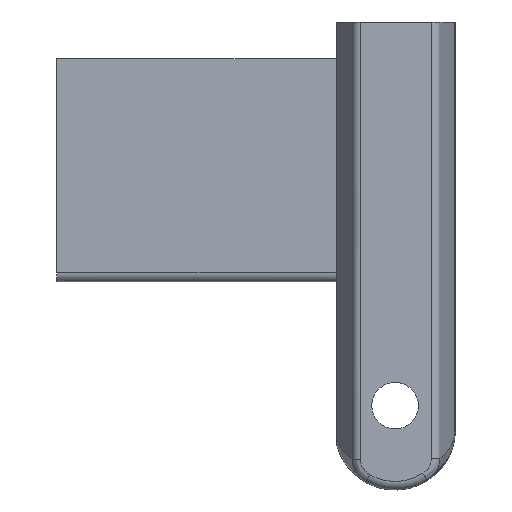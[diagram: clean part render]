
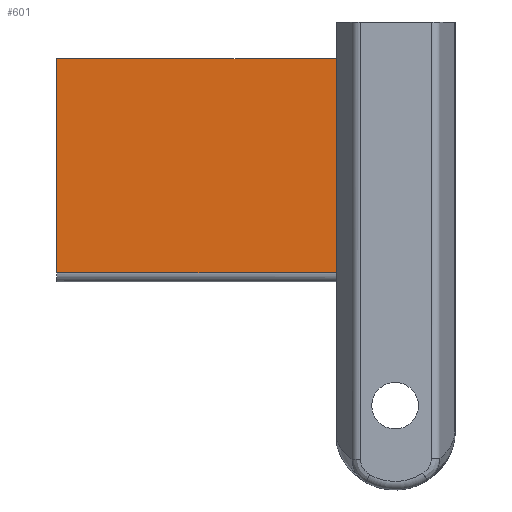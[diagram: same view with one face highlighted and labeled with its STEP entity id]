
A CAD part, front view. The second image highlights one B-rep face of the part: STEP entity #601.
In plain terms, the highlighted planar face has unit normal (0, -1, 0).
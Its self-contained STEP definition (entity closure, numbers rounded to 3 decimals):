
#13 = CARTESIAN_POINT ( 'NONE',  ( -220.232, 17.562, 12.503 ) ) ;
#50 = VECTOR ( 'NONE', #568, 1000. ) ;
#51 = CARTESIAN_POINT ( 'NONE',  ( -227.401, 17.562, -12.057 ) ) ;
#61 = ORIENTED_EDGE ( 'NONE', *, *, #548, .T. ) ;
#78 = CARTESIAN_POINT ( 'NONE',  ( -220.205, 17.562, -4.432 ) ) ;
#81 = DIRECTION ( 'NONE',  ( 0., 0., -1. ) ) ;
#115 = EDGE_CURVE ( 'NONE', #685, #707, #315, .T. ) ;
#133 = EDGE_CURVE ( 'NONE', #310, #685, #245, .T. ) ;
#135 = VERTEX_POINT ( 'NONE', #640 ) ;
#141 = ORIENTED_EDGE ( 'NONE', *, *, #941, .T. ) ;
#143 = EDGE_LOOP ( 'NONE', ( #504, #1199, #1177, #967, #61, #413, #949, #141 ) ) ;
#144 = DIRECTION ( 'NONE',  ( -1., 0., 0. ) ) ;
#245 = LINE ( 'NONE', #470, #500 ) ;
#265 = DIRECTION ( 'NONE',  ( 0., -1., 0. ) ) ;
#273 = CARTESIAN_POINT ( 'NONE',  ( -224.381, 17.562, -5.772 ) ) ;
#309 = CARTESIAN_POINT ( 'NONE',  ( -227.401, 17.562, -17.057 ) ) ;
#310 = VERTEX_POINT ( 'NONE', #770 ) ;
#315 = LINE ( 'NONE', #829, #610 ) ;
#343 = VECTOR ( 'NONE', #497, 1000. ) ;
#357 = AXIS2_PLACEMENT_3D ( 'NONE', #273, #265, #1133 ) ;
#370 = FACE_OUTER_BOUND ( 'NONE', #143, .T. ) ;
#380 = EDGE_CURVE ( 'NONE', #1049, #617, #841, .T. ) ;
#386 = CARTESIAN_POINT ( 'NONE',  ( -252.316, 17.562, -12.057 ) ) ;
#413 = ORIENTED_EDGE ( 'NONE', *, *, #380, .F. ) ;
#427 = LINE ( 'NONE', #78, #607 ) ;
#430 = LINE ( 'NONE', #757, #343 ) ;
#462 = PLANE ( 'NONE',  #357 ) ;
#470 = CARTESIAN_POINT ( 'NONE',  ( -220.232, 17.562, 8.365 ) ) ;
#497 = DIRECTION ( 'NONE',  ( 0., 0., 1. ) ) ;
#500 = VECTOR ( 'NONE', #743, 1000. ) ;
#504 = ORIENTED_EDGE ( 'NONE', *, *, #1169, .F. ) ;
#542 = CARTESIAN_POINT ( 'NONE',  ( -218.007, 17.562, 16.723 ) ) ;
#548 = EDGE_CURVE ( 'NONE', #707, #617, #706, .T. ) ;
#568 = DIRECTION ( 'NONE',  ( 1., 0., 0. ) ) ;
#583 = EDGE_CURVE ( 'NONE', #1030, #310, #1007, .T. ) ;
#601 = ADVANCED_FACE ( 'NONE', ( #370 ), #462, .T. ) ;
#607 = VECTOR ( 'NONE', #81, 1000. ) ;
#610 = VECTOR ( 'NONE', #942, 1000. ) ;
#617 = VERTEX_POINT ( 'NONE', #386 ) ;
#640 = CARTESIAN_POINT ( 'NONE',  ( -220.21, 17.562, -17.057 ) ) ;
#685 = VERTEX_POINT ( 'NONE', #13 ) ;
#706 = LINE ( 'NONE', #1210, #1171 ) ;
#707 = VERTEX_POINT ( 'NONE', #939 ) ;
#714 = CARTESIAN_POINT ( 'NONE',  ( -220.21, 17.562, -12.057 ) ) ;
#743 = DIRECTION ( 'NONE',  ( 0., 0., -1. ) ) ;
#757 = CARTESIAN_POINT ( 'NONE',  ( -220.21, 17.562, -8.363 ) ) ;
#770 = CARTESIAN_POINT ( 'NONE',  ( -220.232, 17.562, 16.723 ) ) ;
#787 = CARTESIAN_POINT ( 'NONE',  ( -220.205, 17.562, -17.057 ) ) ;
#824 = DIRECTION ( 'NONE',  ( -1., 0., 0. ) ) ;
#829 = CARTESIAN_POINT ( 'NONE',  ( -226.214, 17.562, 12.503 ) ) ;
#841 = LINE ( 'NONE', #51, #1078 ) ;
#931 = EDGE_CURVE ( 'NONE', #135, #1049, #430, .T. ) ;
#939 = CARTESIAN_POINT ( 'NONE',  ( -252.316, 17.562, 12.503 ) ) ;
#941 = EDGE_CURVE ( 'NONE', #135, #1100, #1065, .T. ) ;
#942 = DIRECTION ( 'NONE',  ( -1., 0., 0. ) ) ;
#949 = ORIENTED_EDGE ( 'NONE', *, *, #931, .F. ) ;
#967 = ORIENTED_EDGE ( 'NONE', *, *, #115, .T. ) ;
#986 = CARTESIAN_POINT ( 'NONE',  ( -220.205, 17.562, 16.723 ) ) ;
#1007 = LINE ( 'NONE', #542, #1197 ) ;
#1030 = VERTEX_POINT ( 'NONE', #986 ) ;
#1049 = VERTEX_POINT ( 'NONE', #714 ) ;
#1065 = LINE ( 'NONE', #309, #50 ) ;
#1078 = VECTOR ( 'NONE', #144, 1000. ) ;
#1100 = VERTEX_POINT ( 'NONE', #787 ) ;
#1133 = DIRECTION ( 'NONE',  ( 1., 0., 0. ) ) ;
#1169 = EDGE_CURVE ( 'NONE', #1030, #1100, #427, .T. ) ;
#1171 = VECTOR ( 'NONE', #1206, 1000. ) ;
#1177 = ORIENTED_EDGE ( 'NONE', *, *, #133, .T. ) ;
#1197 = VECTOR ( 'NONE', #824, 1000. ) ;
#1199 = ORIENTED_EDGE ( 'NONE', *, *, #583, .T. ) ;
#1206 = DIRECTION ( 'NONE',  ( 0., 0., -1. ) ) ;
#1210 = CARTESIAN_POINT ( 'NONE',  ( -252.316, 17.562, -3.025 ) ) ;
